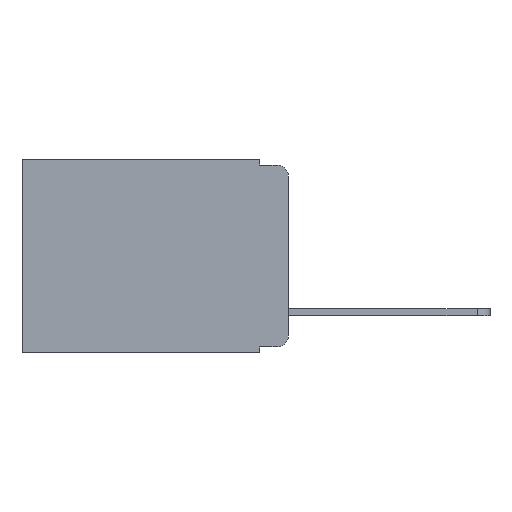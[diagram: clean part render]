
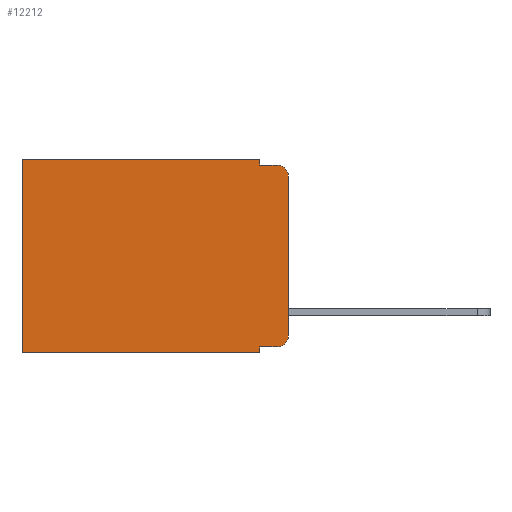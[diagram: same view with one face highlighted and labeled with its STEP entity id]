
A CAD part, left-side view. The second image highlights one B-rep face of the part: STEP entity #12212.
In plain terms, the highlighted planar face has unit normal (-1, 0, 0).
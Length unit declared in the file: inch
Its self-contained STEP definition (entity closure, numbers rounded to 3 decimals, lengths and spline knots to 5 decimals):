
#134 = CIRCLE ( 'NONE', #7223, 0.02 ) ;
#214 = CARTESIAN_POINT ( 'NONE',  ( 0.298, 0.051, -0.333 ) ) ;
#380 = ORIENTED_EDGE ( 'NONE', *, *, #2601, .F. ) ;
#525 = EDGE_CURVE ( 'NONE', #13447, #13566, #10365, .T. ) ;
#598 = ORIENTED_EDGE ( 'NONE', *, *, #7279, .F. ) ;
#852 = CARTESIAN_POINT ( 'NONE',  ( 0.298, 0., 0. ) ) ;
#951 = CARTESIAN_POINT ( 'NONE',  ( 0.298, 0.051, 0. ) ) ;
#1023 = DIRECTION ( 'NONE',  ( 0., 0., -1. ) ) ;
#1248 = VERTEX_POINT ( 'NONE', #11523 ) ;
#1289 = ORIENTED_EDGE ( 'NONE', *, *, #525, .T. ) ;
#1858 = VECTOR ( 'NONE', #9026, 39.37008 ) ;
#2601 = EDGE_CURVE ( 'NONE', #13259, #15265, #5686, .T. ) ;
#2602 = VECTOR ( 'NONE', #16890, 39.37008 ) ;
#2621 = CARTESIAN_POINT ( 'NONE',  ( 0.298, 0.02, -0.03 ) ) ;
#2712 = VECTOR ( 'NONE', #4740, 39.37008 ) ;
#2738 = CARTESIAN_POINT ( 'NONE',  ( 0.298, 0., -0.343 ) ) ;
#3161 = DIRECTION ( 'NONE',  ( 0., 0., -1. ) ) ;
#3865 = PLANE ( 'NONE',  #12939 ) ;
#4020 = VECTOR ( 'NONE', #9060, 39.37008 ) ;
#4055 = DIRECTION ( 'NONE',  ( 0., 0., -1. ) ) ;
#4244 = CARTESIAN_POINT ( 'NONE',  ( 0.298, 0.051, -0.01 ) ) ;
#4461 = LINE ( 'NONE', #852, #11128 ) ;
#4740 = DIRECTION ( 'NONE',  ( 0., -1., 0. ) ) ;
#4885 = ORIENTED_EDGE ( 'NONE', *, *, #11841, .T. ) ;
#4952 = LINE ( 'NONE', #12125, #11570 ) ;
#5490 = EDGE_CURVE ( 'NONE', #13259, #12510, #4461, .T. ) ;
#5621 = DIRECTION ( 'NONE',  ( 0., 0., -1. ) ) ;
#5686 = LINE ( 'NONE', #951, #1858 ) ;
#5764 = ORIENTED_EDGE ( 'NONE', *, *, #5490, .T. ) ;
#6005 = CARTESIAN_POINT ( 'NONE',  ( 0.298, 0., -0.03 ) ) ;
#6382 = LINE ( 'NONE', #9928, #10298 ) ;
#6383 = VERTEX_POINT ( 'NONE', #6005 ) ;
#7223 = AXIS2_PLACEMENT_3D ( 'NONE', #2621, #12011, #4055 ) ;
#7279 = EDGE_CURVE ( 'NONE', #6383, #12548, #13222, .T. ) ;
#7286 = VERTEX_POINT ( 'NONE', #16169 ) ;
#7323 = CARTESIAN_POINT ( 'NONE',  ( 0.298, 0.02, -0.313 ) ) ;
#7527 = EDGE_LOOP ( 'NONE', ( #598, #4885, #14256, #380, #5764, #13842, #15034, #12878, #1289, #16212 ) ) ;
#7719 = VERTEX_POINT ( 'NONE', #14514 ) ;
#8212 = DIRECTION ( 'NONE',  ( 0., 1., 0. ) ) ;
#8629 = DIRECTION ( 'NONE',  ( 0., 0., -1. ) ) ;
#8688 = CARTESIAN_POINT ( 'NONE',  ( 0.298, 0.473, 0. ) ) ;
#9026 = DIRECTION ( 'NONE',  ( 0., 0., -1. ) ) ;
#9060 = DIRECTION ( 'NONE',  ( 0., -1., 0. ) ) ;
#9324 = DIRECTION ( 'NONE',  ( 1., 0., 0. ) ) ;
#9683 = LINE ( 'NONE', #2738, #10097 ) ;
#9928 = CARTESIAN_POINT ( 'NONE',  ( 0.298, 0.051, 0. ) ) ;
#10041 = EDGE_CURVE ( 'NONE', #12510, #1248, #4952, .T. ) ;
#10076 = CIRCLE ( 'NONE', #10091, 0.02 ) ;
#10091 = AXIS2_PLACEMENT_3D ( 'NONE', #7323, #16217, #8629 ) ;
#10097 = VECTOR ( 'NONE', #8212, 39.37008 ) ;
#10223 = CARTESIAN_POINT ( 'NONE',  ( 0.298, 0.051, 0. ) ) ;
#10298 = VECTOR ( 'NONE', #3161, 39.37008 ) ;
#10365 = LINE ( 'NONE', #214, #2712 ) ;
#11017 = EDGE_CURVE ( 'NONE', #15265, #7286, #14479, .T. ) ;
#11090 = FACE_OUTER_BOUND ( 'NONE', #7527, .T. ) ;
#11128 = VECTOR ( 'NONE', #11241, 39.37008 ) ;
#11241 = DIRECTION ( 'NONE',  ( 0., 1., 0. ) ) ;
#11364 = CARTESIAN_POINT ( 'NONE',  ( 0.298, 0., -0.313 ) ) ;
#11523 = CARTESIAN_POINT ( 'NONE',  ( 0.298, 0.473, -0.343 ) ) ;
#11544 = CARTESIAN_POINT ( 'NONE',  ( 0.298, 0., 0. ) ) ;
#11570 = VECTOR ( 'NONE', #5621, 39.37008 ) ;
#11841 = EDGE_CURVE ( 'NONE', #6383, #7286, #134, .T. ) ;
#11858 = CARTESIAN_POINT ( 'NONE',  ( 0.298, 0., 0. ) ) ;
#12011 = DIRECTION ( 'NONE',  ( -1., 0., 0. ) ) ;
#12125 = CARTESIAN_POINT ( 'NONE',  ( 0.298, 0.473, 0. ) ) ;
#12212 = ADVANCED_FACE ( 'NONE', ( #11090 ), #3865, .F. ) ;
#12462 = EDGE_CURVE ( 'NONE', #13566, #12548, #10076, .T. ) ;
#12510 = VERTEX_POINT ( 'NONE', #8688 ) ;
#12548 = VERTEX_POINT ( 'NONE', #11364 ) ;
#12878 = ORIENTED_EDGE ( 'NONE', *, *, #16039, .F. ) ;
#12939 = AXIS2_PLACEMENT_3D ( 'NONE', #11858, #9324, #1023 ) ;
#13222 = LINE ( 'NONE', #11544, #2602 ) ;
#13259 = VERTEX_POINT ( 'NONE', #10223 ) ;
#13447 = VERTEX_POINT ( 'NONE', #16886 ) ;
#13566 = VERTEX_POINT ( 'NONE', #15863 ) ;
#13842 = ORIENTED_EDGE ( 'NONE', *, *, #10041, .T. ) ;
#14256 = ORIENTED_EDGE ( 'NONE', *, *, #11017, .F. ) ;
#14479 = LINE ( 'NONE', #15367, #4020 ) ;
#14514 = CARTESIAN_POINT ( 'NONE',  ( 0.298, 0.051, -0.343 ) ) ;
#15034 = ORIENTED_EDGE ( 'NONE', *, *, #15843, .F. ) ;
#15265 = VERTEX_POINT ( 'NONE', #4244 ) ;
#15367 = CARTESIAN_POINT ( 'NONE',  ( 0.298, 0.051, -0.01 ) ) ;
#15843 = EDGE_CURVE ( 'NONE', #7719, #1248, #9683, .T. ) ;
#15863 = CARTESIAN_POINT ( 'NONE',  ( 0.298, 0.02, -0.333 ) ) ;
#16039 = EDGE_CURVE ( 'NONE', #13447, #7719, #6382, .T. ) ;
#16169 = CARTESIAN_POINT ( 'NONE',  ( 0.298, 0.02, -0.01 ) ) ;
#16212 = ORIENTED_EDGE ( 'NONE', *, *, #12462, .T. ) ;
#16217 = DIRECTION ( 'NONE',  ( -1., 0., 0. ) ) ;
#16886 = CARTESIAN_POINT ( 'NONE',  ( 0.298, 0.051, -0.333 ) ) ;
#16890 = DIRECTION ( 'NONE',  ( 0., 0., -1. ) ) ;
